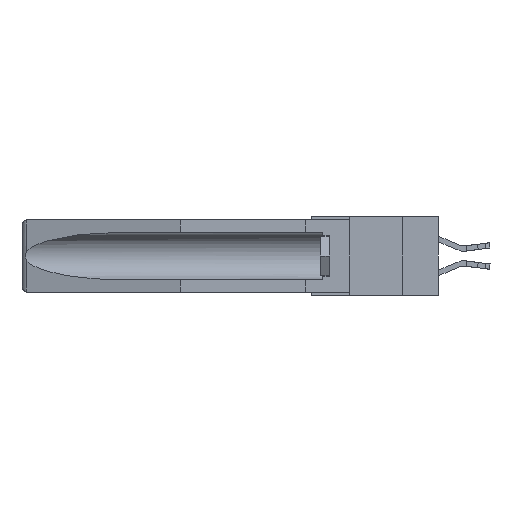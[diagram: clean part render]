
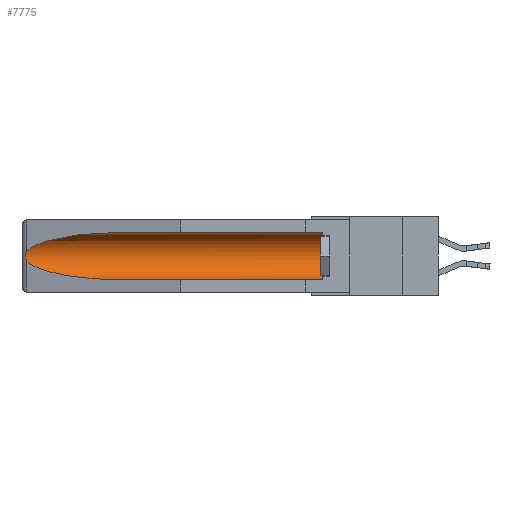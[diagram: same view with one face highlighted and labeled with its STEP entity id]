
A CAD part, left-side view. The second image highlights one B-rep face of the part: STEP entity #7775.
In plain terms, the highlighted cylindrical face has radius 2.857 mm (diameter 5.715 mm), a partial arc.
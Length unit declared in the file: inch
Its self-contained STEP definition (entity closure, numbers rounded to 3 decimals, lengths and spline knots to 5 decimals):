
#74 = CARTESIAN_POINT ( 'NONE',  ( 0.155, -0.30754, -0.059 ) ) ;
#330 = CARTESIAN_POINT ( 'NONE',  ( 0.155, 0.126, -0.1715 ) ) ;
#449 = CARTESIAN_POINT ( 'NONE',  ( 0.155, 0.126, -0.059 ) ) ;
#512 = ORIENTED_EDGE ( 'NONE', *, *, #13869, .T. ) ;
#702 = CARTESIAN_POINT ( 'NONE',  ( 0.155, 1.07973, -0.284 ) ) ;
#781 = CARTESIAN_POINT ( 'NONE',  ( 0.26537, 1.52718, -0.19328 ) ) ;
#1100 = VERTEX_POINT ( 'NONE', #8736 ) ;
#1395 = CARTESIAN_POINT ( 'NONE',  ( 0.155, -0.30754, -0.284 ) ) ;
#1503 = LINE ( 'NONE', #1395, #14450 ) ;
#2322 = CARTESIAN_POINT ( 'NONE',  ( 0.26537, 1.52718, -0.14972 ) ) ;
#2371 = ORIENTED_EDGE ( 'NONE', *, *, #3204, .T. ) ;
#2451 = CARTESIAN_POINT ( 'NONE',  ( 0.2673, 1.5327, -0.16383 ) ) ;
#2532 = CARTESIAN_POINT ( 'NONE',  ( 0.2675, 1.53308, -0.17534 ) ) ;
#2916 = ORIENTED_EDGE ( 'NONE', *, *, #4621, .T. ) ;
#3021 = CARTESIAN_POINT ( 'NONE',  ( 0.155, 1.07973, -0.059 ) ) ;
#3204 = EDGE_CURVE ( 'NONE', #11982, #20578, #21619, .T. ) ;
#3734 = AXIS2_PLACEMENT_3D ( 'NONE', #330, #15796, #12160 ) ;
#3873 =( BOUNDED_CURVE ( )  B_SPLINE_CURVE ( 3, ( #3021, #13226, #13517, #8314 ),
 .UNSPECIFIED., .F., .F. ) 
 B_SPLINE_CURVE_WITH_KNOTS ( ( 4, 4 ),
 ( 4.71239, 6.08839 ),
 .UNSPECIFIED. ) 
 CURVE ( )  GEOMETRIC_REPRESENTATION_ITEM ( )  RATIONAL_B_SPLINE_CURVE ( ( 1., 0.848, 0.848, 1. ) ) 
 REPRESENTATION_ITEM ( '' )  );
#4238 = CARTESIAN_POINT ( 'NONE',  ( 0.2673, 1.53269, -0.17917 ) ) ;
#4621 = EDGE_CURVE ( 'NONE', #1100, #11982, #3873, .T. ) ;
#4957 =( BOUNDED_CURVE ( )  B_SPLINE_CURVE ( 3, ( #781, #17576, #10659, #702 ),
 .UNSPECIFIED., .F., .F. ) 
 B_SPLINE_CURVE_WITH_KNOTS ( ( 4, 4 ),
 ( 0.1948, 1.5708 ),
 .UNSPECIFIED. ) 
 CURVE ( )  GEOMETRIC_REPRESENTATION_ITEM ( )  RATIONAL_B_SPLINE_CURVE ( ( 1., 0.848, 0.848, 1. ) ) 
 REPRESENTATION_ITEM ( '' )  );
#5960 = VERTEX_POINT ( 'NONE', #13503 ) ;
#6969 = CARTESIAN_POINT ( 'NONE',  ( 0.155, -0.30754, -0.1715 ) ) ;
#7118 = DIRECTION ( 'NONE',  ( 0., 0., 1. ) ) ;
#7775 = ADVANCED_FACE ( 'NONE', ( #17383 ), #8798, .F. ) ;
#8095 = EDGE_CURVE ( 'NONE', #20745, #5960, #1503, .T. ) ;
#8314 = CARTESIAN_POINT ( 'NONE',  ( 0.26537, 1.52718, -0.14972 ) ) ;
#8736 = CARTESIAN_POINT ( 'NONE',  ( 0.155, 1.07973, -0.059 ) ) ;
#8798 = CYLINDRICAL_SURFACE ( 'NONE', #11464, 0.1125 ) ;
#9002 = EDGE_CURVE ( 'NONE', #20745, #11649, #14134, .T. ) ;
#9096 = CARTESIAN_POINT ( 'NONE',  ( 0.26654, 1.53092, -0.15636 ) ) ;
#10100 = DIRECTION ( 'NONE',  ( 0., 1., 0. ) ) ;
#10507 = ORIENTED_EDGE ( 'NONE', *, *, #8095, .F. ) ;
#10659 = CARTESIAN_POINT ( 'NONE',  ( 0.21114, 1.30732, -0.284 ) ) ;
#11151 = CARTESIAN_POINT ( 'NONE',  ( 0.26655, 1.53094, -0.18657 ) ) ;
#11464 = AXIS2_PLACEMENT_3D ( 'NONE', #6969, #17117, #7118 ) ;
#11635 = ORIENTED_EDGE ( 'NONE', *, *, #16184, .T. ) ;
#11649 = VERTEX_POINT ( 'NONE', #449 ) ;
#11982 = VERTEX_POINT ( 'NONE', #13930 ) ;
#12160 = DIRECTION ( 'NONE',  ( 0., 0., 1. ) ) ;
#13226 = CARTESIAN_POINT ( 'NONE',  ( 0.21114, 1.30732, -0.059 ) ) ;
#13503 = CARTESIAN_POINT ( 'NONE',  ( 0.155, 1.07973, -0.284 ) ) ;
#13517 = CARTESIAN_POINT ( 'NONE',  ( 0.25451, 1.48313, -0.09465 ) ) ;
#13869 = EDGE_CURVE ( 'NONE', #20578, #5960, #4957, .T. ) ;
#13930 = CARTESIAN_POINT ( 'NONE',  ( 0.26537, 1.52718, -0.14972 ) ) ;
#14134 = CIRCLE ( 'NONE', #3734, 0.1125 ) ;
#14162 = EDGE_LOOP ( 'NONE', ( #2916, #2371, #512, #10507, #19133, #11635 ) ) ;
#14450 = VECTOR ( 'NONE', #14825, 39.37008 ) ;
#14825 = DIRECTION ( 'NONE',  ( 0., 1., 0. ) ) ;
#15796 = DIRECTION ( 'NONE',  ( 0., -1., 0. ) ) ;
#15849 = CARTESIAN_POINT ( 'NONE',  ( 0.26597, 1.52961, -0.15275 ) ) ;
#16184 = EDGE_CURVE ( 'NONE', #11649, #1100, #16384, .T. ) ;
#16384 = LINE ( 'NONE', #74, #20121 ) ;
#17117 = DIRECTION ( 'NONE',  ( 0., 1., 0. ) ) ;
#17383 = FACE_OUTER_BOUND ( 'NONE', #14162, .T. ) ;
#17576 = CARTESIAN_POINT ( 'NONE',  ( 0.25451, 1.48313, -0.24835 ) ) ;
#18073 = CARTESIAN_POINT ( 'NONE',  ( 0.26537, 1.52718, -0.19328 ) ) ;
#18534 = CARTESIAN_POINT ( 'NONE',  ( 0.26597, 1.5296, -0.19026 ) ) ;
#19133 = ORIENTED_EDGE ( 'NONE', *, *, #9002, .T. ) ;
#19537 = CARTESIAN_POINT ( 'NONE',  ( 0.26537, 1.52718, -0.19328 ) ) ;
#20121 = VECTOR ( 'NONE', #10100, 39.37008 ) ;
#20578 = VERTEX_POINT ( 'NONE', #19537 ) ;
#20745 = VERTEX_POINT ( 'NONE', #21590 ) ;
#21109 = CARTESIAN_POINT ( 'NONE',  ( 0.2675, 1.53308, -0.16763 ) ) ;
#21590 = CARTESIAN_POINT ( 'NONE',  ( 0.155, 0.126, -0.284 ) ) ;
#21619 = B_SPLINE_CURVE_WITH_KNOTS ( 'NONE', 3,
 ( #2322, #15849, #9096, #2451, #21109, #2532, #4238, #11151, #18534, #18073 ),
 .UNSPECIFIED., .F., .F.,
 ( 4, 2, 2, 2, 4 ),
 ( 0., 0.00029, 0.00058, 0.00087, 0.00117 ),
 .UNSPECIFIED. ) ;
